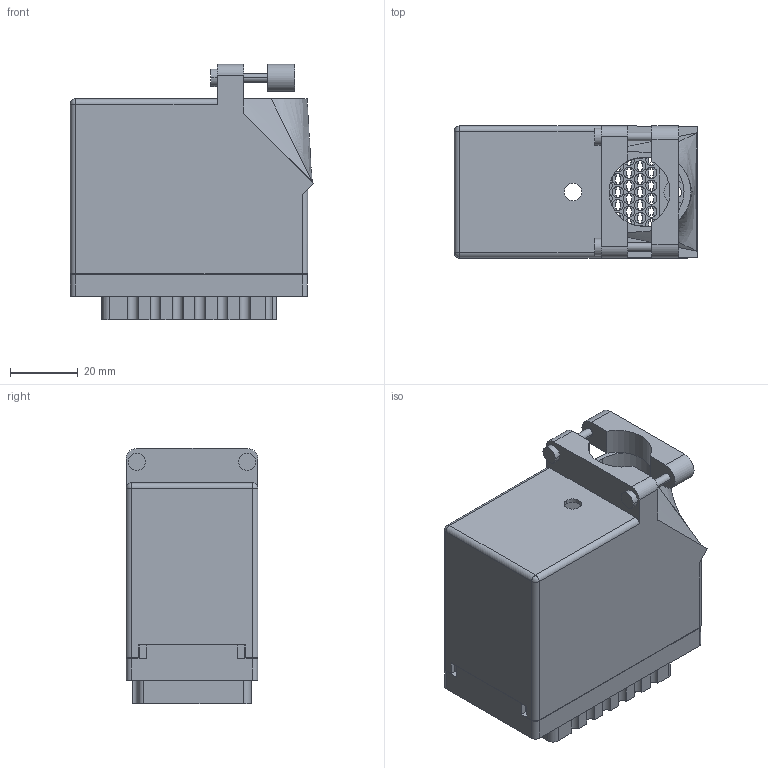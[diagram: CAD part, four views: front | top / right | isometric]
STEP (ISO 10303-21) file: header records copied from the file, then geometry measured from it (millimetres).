
FILE_DESCRIPTION (( 'STEP AP203' ), '1' );
FILE_NAME ('516-120-000-410.STEP', '2020-03-06T23:56:07', ( '' ), ( '' ), 'SwSTEP 2.0', 'SolidWorks 2016', '' );
FILE_SCHEMA (( 'CONFIG_CONTROL_DESIGN' ));
Length unit declared in the file: inch
Products named in the file (3): 516-230-001_Plastic - 120 Top Entry; 516-120-000-410; 516 Part Receptacle_120
Assembly tree (2 placements, depth 2):
  516-120-000-410
    516 Part Receptacle_120
    516-230-001_Plastic - 120 Top Entry
Bounding box: 71.77 x 38.86 x 75.21 mm (x, y, z)
Volume: 47445.7 mm3; surface area: 65132.7 mm2
Topology: 2 solids, 2 shells, 2557 faces, 7588 edges, 5054 vertices
Faces by surface type: plane 1828, cylinder 722, bspline 3, cone 2, sphere 2
Entity records: 86554 total; most frequent: CARTESIAN_POINT 15303, ORIENTED_EDGE 15172, DIRECTION 14623, EDGE_CURVE 7586, VECTOR 5659, LINE 5659, VERTEX_POINT 5054, AXIS2_PLACEMENT_3D 4482
